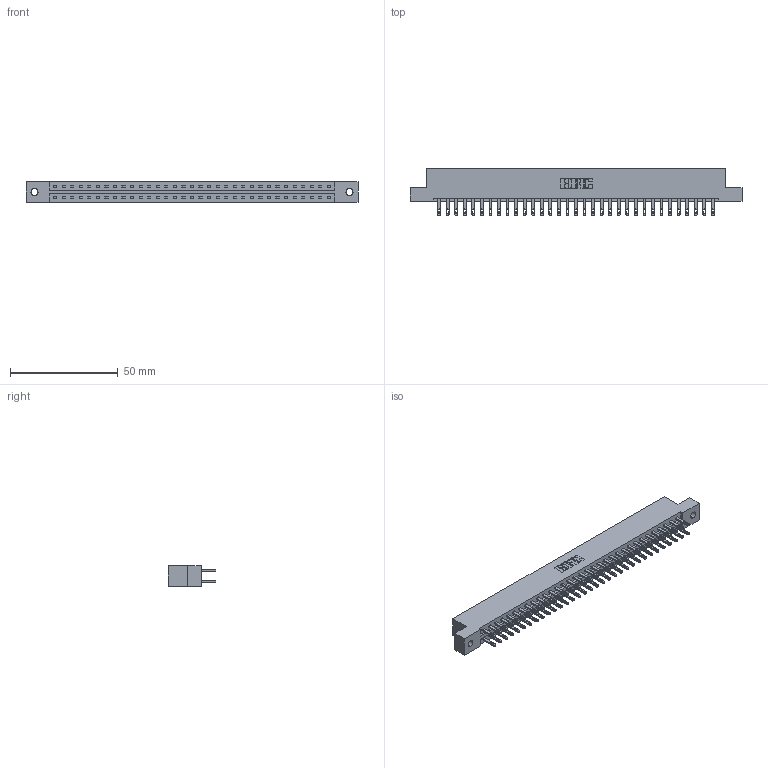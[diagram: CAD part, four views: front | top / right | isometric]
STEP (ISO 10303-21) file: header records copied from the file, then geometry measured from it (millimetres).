
FILE_DESCRIPTION (( 'STEP AP203' ), '1' );
FILE_NAME ('887-066-500-202.STEP', '2020-09-21T02:42:47', ( '' ), ( '' ), 'SwSTEP 2.0', 'SolidWorks 2020', '' );
FILE_SCHEMA (( 'CONFIG_CONTROL_DESIGN' ));
Length unit declared in the file: inch
Products named in the file (3): 345-292-001_345-293-100; 887-066-500-202; 837 Part_Flush Mounting Lugs - 0.128 Dia
Assembly tree (67 placements, depth 2):
  887-066-500-202
    837 Part_Flush Mounting Lugs - 0.128 Dia
    345-292-001_345-293-100  x66
Bounding box: 153.77 x 21.85 x 9.4 mm (x, y, z)
Volume: 16250.9 mm3; surface area: 18743.8 mm2
Topology: 67 solids, 67 shells, 3414 faces, 10409 edges, 6938 vertices
Faces by surface type: plane 2182, cylinder 1232
Entity records: 26683 total; most frequent: CARTESIAN_POINT 4502, ORIENTED_EDGE 4438, DIRECTION 3847, EDGE_CURVE 2219, LINE 2087, VECTOR 2087, VERTEX_POINT 1478, AXIS2_PLACEMENT_3D 880
